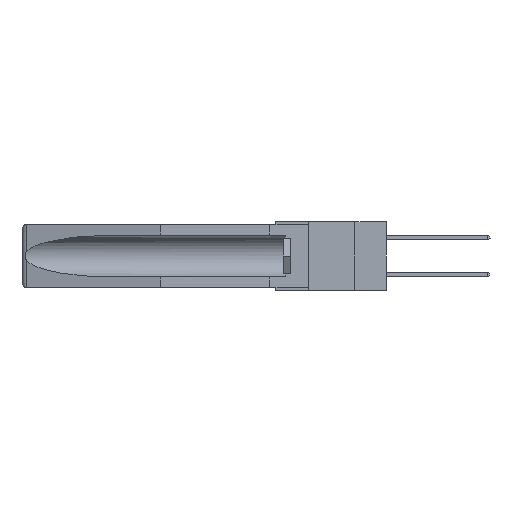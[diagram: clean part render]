
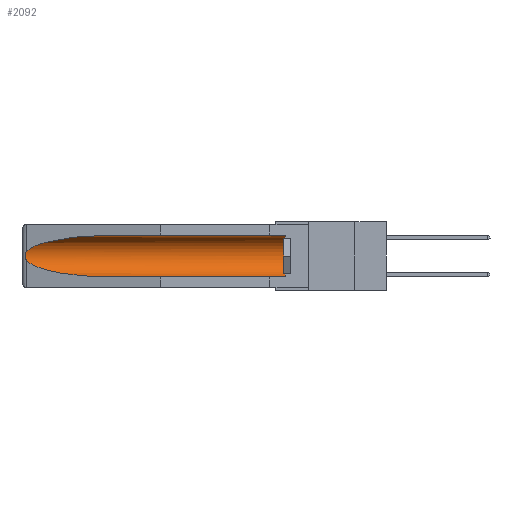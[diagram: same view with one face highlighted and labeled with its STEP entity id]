
A CAD part, left-side view. The second image highlights one B-rep face of the part: STEP entity #2092.
In plain terms, the highlighted cylindrical face has radius 2.857 mm (diameter 5.715 mm), a partial arc.
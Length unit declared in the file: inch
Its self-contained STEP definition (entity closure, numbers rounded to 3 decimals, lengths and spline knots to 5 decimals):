
#123 = CARTESIAN_POINT ( 'NONE',  ( 0.155, 1.07973, -0.059 ) ) ;
#165 = ORIENTED_EDGE ( 'NONE', *, *, #4726, .T. ) ;
#804 = VERTEX_POINT ( 'NONE', #2912 ) ;
#1635 = CARTESIAN_POINT ( 'NONE',  ( 0.26537, 1.52718, -0.14972 ) ) ;
#1665 = DIRECTION ( 'NONE',  ( 0., 1., 0. ) ) ;
#2092 = ADVANCED_FACE ( 'NONE', ( #3316 ), #7042, .F. ) ;
#2229 = CARTESIAN_POINT ( 'NONE',  ( 0.26655, 1.53094, -0.18657 ) ) ;
#2912 = CARTESIAN_POINT ( 'NONE',  ( 0.155, 0.126, -0.059 ) ) ;
#2992 = ORIENTED_EDGE ( 'NONE', *, *, #16093, .T. ) ;
#3038 = EDGE_CURVE ( 'NONE', #13037, #13519, #18351, .T. ) ;
#3316 = FACE_OUTER_BOUND ( 'NONE', #3639, .T. ) ;
#3503 = EDGE_CURVE ( 'NONE', #13587, #16500, #14982, .T. ) ;
#3639 = EDGE_LOOP ( 'NONE', ( #10275, #165, #11269, #6411, #18453, #2992 ) ) ;
#4055 = LINE ( 'NONE', #13077, #11643 ) ;
#4398 = CARTESIAN_POINT ( 'NONE',  ( 0.25451, 1.48313, -0.09465 ) ) ;
#4704 = CARTESIAN_POINT ( 'NONE',  ( 0.21114, 1.30732, -0.284 ) ) ;
#4726 = EDGE_CURVE ( 'NONE', #13519, #13587, #12591, .T. ) ;
#5118 = VERTEX_POINT ( 'NONE', #8522 ) ;
#5245 = DIRECTION ( 'NONE',  ( 0., -1., 0. ) ) ;
#6212 = EDGE_CURVE ( 'NONE', #5118, #16500, #4055, .T. ) ;
#6411 = ORIENTED_EDGE ( 'NONE', *, *, #6212, .F. ) ;
#6573 = CIRCLE ( 'NONE', #8342, 0.1125 ) ;
#6838 = CARTESIAN_POINT ( 'NONE',  ( 0.26597, 1.5296, -0.19026 ) ) ;
#7042 = CYLINDRICAL_SURFACE ( 'NONE', #15847, 0.1125 ) ;
#7351 = DIRECTION ( 'NONE',  ( 0., 1., 0. ) ) ;
#7718 = DIRECTION ( 'NONE',  ( 0., 1., 0. ) ) ;
#7828 = DIRECTION ( 'NONE',  ( 0., 0., 1. ) ) ;
#8138 = CARTESIAN_POINT ( 'NONE',  ( 0.155, 0.126, -0.1715 ) ) ;
#8342 = AXIS2_PLACEMENT_3D ( 'NONE', #8138, #5245, #16747 ) ;
#8522 = CARTESIAN_POINT ( 'NONE',  ( 0.155, 0.126, -0.284 ) ) ;
#8663 = LINE ( 'NONE', #9147, #10696 ) ;
#8865 = CARTESIAN_POINT ( 'NONE',  ( 0.155, -0.30754, -0.1715 ) ) ;
#9147 = CARTESIAN_POINT ( 'NONE',  ( 0.155, -0.30754, -0.059 ) ) ;
#9631 = CARTESIAN_POINT ( 'NONE',  ( 0.2673, 1.5327, -0.16383 ) ) ;
#10232 = CARTESIAN_POINT ( 'NONE',  ( 0.21114, 1.30732, -0.059 ) ) ;
#10275 = ORIENTED_EDGE ( 'NONE', *, *, #3038, .T. ) ;
#10534 = CARTESIAN_POINT ( 'NONE',  ( 0.155, 1.07973, -0.284 ) ) ;
#10696 = VECTOR ( 'NONE', #1665, 39.37008 ) ;
#11018 = CARTESIAN_POINT ( 'NONE',  ( 0.2673, 1.53269, -0.17917 ) ) ;
#11140 = CARTESIAN_POINT ( 'NONE',  ( 0.2675, 1.53308, -0.17534 ) ) ;
#11269 = ORIENTED_EDGE ( 'NONE', *, *, #3503, .T. ) ;
#11643 = VECTOR ( 'NONE', #7351, 39.37008 ) ;
#11895 = CARTESIAN_POINT ( 'NONE',  ( 0.26537, 1.52718, -0.14972 ) ) ;
#12591 = B_SPLINE_CURVE_WITH_KNOTS ( 'NONE', 3,
 ( #17004, #15389, #18521, #9631, #15580, #11140, #11018, #2229, #6838, #15448 ),
 .UNSPECIFIED., .F., .F.,
 ( 4, 2, 2, 2, 4 ),
 ( 0., 0.00029, 0.00058, 0.00087, 0.00117 ),
 .UNSPECIFIED. ) ;
#13037 = VERTEX_POINT ( 'NONE', #15711 ) ;
#13077 = CARTESIAN_POINT ( 'NONE',  ( 0.155, -0.30754, -0.284 ) ) ;
#13519 = VERTEX_POINT ( 'NONE', #1635 ) ;
#13587 = VERTEX_POINT ( 'NONE', #19024 ) ;
#14024 = EDGE_CURVE ( 'NONE', #5118, #804, #6573, .T. ) ;
#14398 = CARTESIAN_POINT ( 'NONE',  ( 0.155, 1.07973, -0.284 ) ) ;
#14982 =( BOUNDED_CURVE ( )  B_SPLINE_CURVE ( 3, ( #16512, #16448, #4704, #10534 ),
 .UNSPECIFIED., .F., .F. ) 
 B_SPLINE_CURVE_WITH_KNOTS ( ( 4, 4 ),
 ( 0.1948, 1.5708 ),
 .UNSPECIFIED. ) 
 CURVE ( )  GEOMETRIC_REPRESENTATION_ITEM ( )  RATIONAL_B_SPLINE_CURVE ( ( 1., 0.848, 0.848, 1. ) ) 
 REPRESENTATION_ITEM ( '' )  );
#15389 = CARTESIAN_POINT ( 'NONE',  ( 0.26597, 1.52961, -0.15275 ) ) ;
#15448 = CARTESIAN_POINT ( 'NONE',  ( 0.26537, 1.52718, -0.19328 ) ) ;
#15580 = CARTESIAN_POINT ( 'NONE',  ( 0.2675, 1.53308, -0.16763 ) ) ;
#15711 = CARTESIAN_POINT ( 'NONE',  ( 0.155, 1.07973, -0.059 ) ) ;
#15847 = AXIS2_PLACEMENT_3D ( 'NONE', #8865, #7718, #7828 ) ;
#16093 = EDGE_CURVE ( 'NONE', #804, #13037, #8663, .T. ) ;
#16448 = CARTESIAN_POINT ( 'NONE',  ( 0.25451, 1.48313, -0.24835 ) ) ;
#16500 = VERTEX_POINT ( 'NONE', #14398 ) ;
#16512 = CARTESIAN_POINT ( 'NONE',  ( 0.26537, 1.52718, -0.19328 ) ) ;
#16747 = DIRECTION ( 'NONE',  ( 0., 0., 1. ) ) ;
#17004 = CARTESIAN_POINT ( 'NONE',  ( 0.26537, 1.52718, -0.14972 ) ) ;
#18351 =( BOUNDED_CURVE ( )  B_SPLINE_CURVE ( 3, ( #123, #10232, #4398, #11895 ),
 .UNSPECIFIED., .F., .F. ) 
 B_SPLINE_CURVE_WITH_KNOTS ( ( 4, 4 ),
 ( 4.71239, 6.08839 ),
 .UNSPECIFIED. ) 
 CURVE ( )  GEOMETRIC_REPRESENTATION_ITEM ( )  RATIONAL_B_SPLINE_CURVE ( ( 1., 0.848, 0.848, 1. ) ) 
 REPRESENTATION_ITEM ( '' )  );
#18453 = ORIENTED_EDGE ( 'NONE', *, *, #14024, .T. ) ;
#18521 = CARTESIAN_POINT ( 'NONE',  ( 0.26654, 1.53092, -0.15636 ) ) ;
#19024 = CARTESIAN_POINT ( 'NONE',  ( 0.26537, 1.52718, -0.19328 ) ) ;
